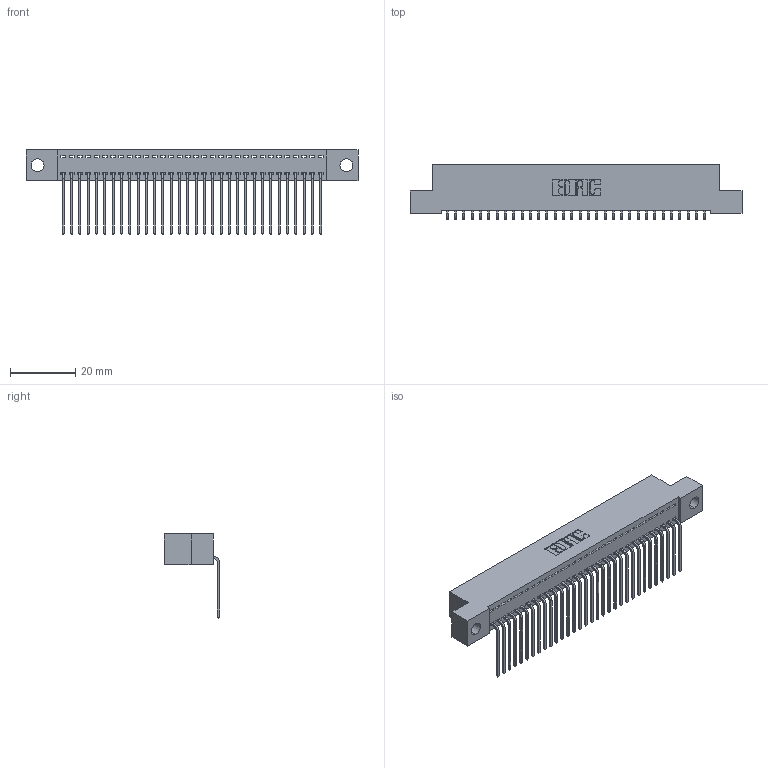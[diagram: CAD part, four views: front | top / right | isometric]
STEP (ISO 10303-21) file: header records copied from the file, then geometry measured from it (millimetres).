
FILE_DESCRIPTION (( 'STEP AP203' ), '1' );
FILE_NAME ('392-032-559-104.STEP', '2019-10-07T15:01:24', ( '' ), ( '' ), 'SwSTEP 2.0', 'SolidWorks 2016', '' );
FILE_SCHEMA (( 'CONFIG_CONTROL_DESIGN' ));
Length unit declared in the file: inch
Products named in the file (3): 342 Part_.156 TH; 345-292-001_558 559 Tail - 1; 392-032-559-104
Assembly tree (33 placements, depth 2):
  392-032-559-104
    342 Part_.156 TH
    345-292-001_558 559 Tail - 1  x32
Bounding box: 101.6 x 16.83 x 25.78 mm (x, y, z)
Volume: 8891 mm3; surface area: 13293.7 mm2
Topology: 33 solids, 33 shells, 2030 faces, 6123 edges, 4038 vertices
Faces by surface type: plane 1474, cylinder 556
Entity records: 20811 total; most frequent: CARTESIAN_POINT 3598, ORIENTED_EDGE 3566, DIRECTION 3055, EDGE_CURVE 1783, LINE 1655, VECTOR 1655, VERTEX_POINT 1186, AXIS2_PLACEMENT_3D 700
